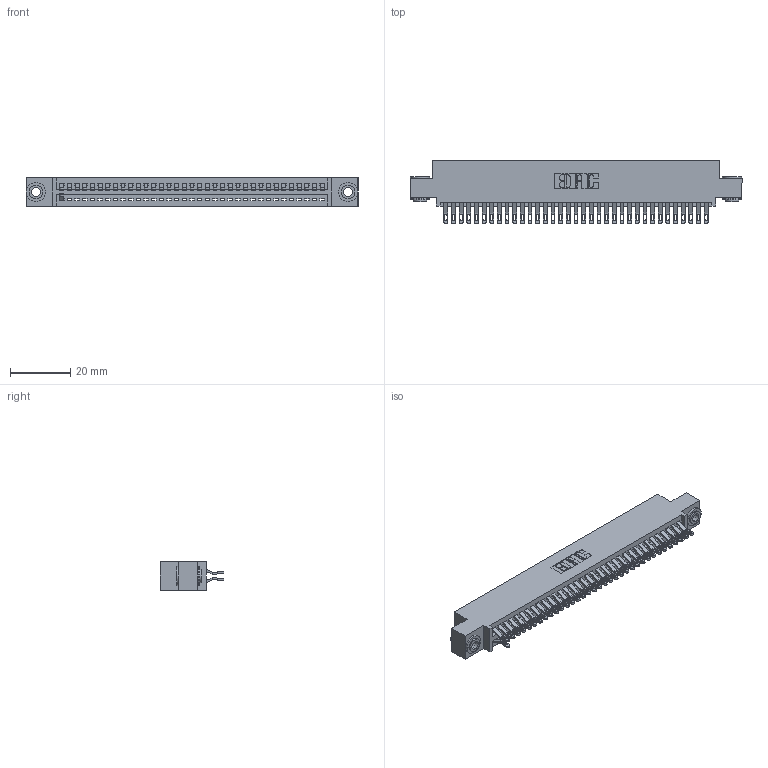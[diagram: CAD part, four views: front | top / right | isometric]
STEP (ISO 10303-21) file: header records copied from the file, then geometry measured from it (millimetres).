
FILE_DESCRIPTION (( 'STEP AP203' ), '1' );
FILE_NAME ('395-070-555-503.STEP', '2018-11-27T00:16:11', ( '' ), ( '' ), 'SwSTEP 2.0', 'SolidWorks 2016', '' );
FILE_SCHEMA (( 'CONFIG_CONTROL_DESIGN' ));
Length unit declared in the file: inch
Products named in the file (4): 345-250-002_345-250-002-102; 345 Part_0.110 Offset - 0.156 Dia-TH; 395-070-555-503; 345-292-001_555 Tail
Assembly tree (39 placements, depth 2):
  395-070-555-503
    345 Part_0.110 Offset - 0.156 Dia-TH
    345-292-001_555 Tail  x36
    345-250-002_345-250-002-102  x2
Bounding box: 110.11 x 21.13 x 9.4 mm (x, y, z)
Volume: 10375.1 mm3; surface area: 14125.6 mm2
Topology: 39 solids, 39 shells, 2456 faces, 7719 edges, 5142 vertices
Faces by surface type: plane 1448, cylinder 1000, cone 8
Entity records: 28424 total; most frequent: CARTESIAN_POINT 4931, ORIENTED_EDGE 4862, DIRECTION 4317, EDGE_CURVE 2431, LINE 2115, VECTOR 2115, VERTEX_POINT 1618, AXIS2_PLACEMENT_3D 1101
